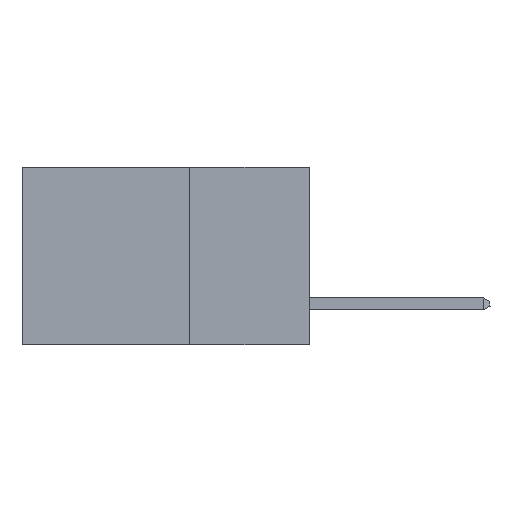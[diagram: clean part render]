
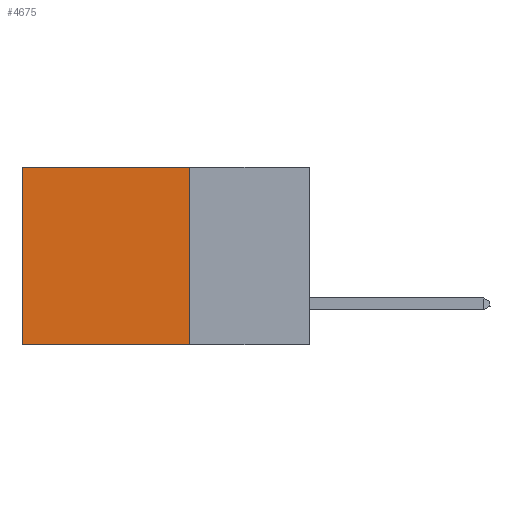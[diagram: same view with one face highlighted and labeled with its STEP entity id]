
A CAD part, left-side view. The second image highlights one B-rep face of the part: STEP entity #4675.
In plain terms, the highlighted planar face has unit normal (-1, 0, 0).
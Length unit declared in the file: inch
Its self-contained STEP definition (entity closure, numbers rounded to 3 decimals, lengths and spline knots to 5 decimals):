
#105 = EDGE_CURVE ( 'NONE', #2544, #1523, #12002, .T. ) ;
#323 = LINE ( 'NONE', #5854, #1986 ) ;
#518 = LINE ( 'NONE', #4223, #8856 ) ;
#544 = DIRECTION ( 'NONE',  ( 0., 1., 0. ) ) ;
#1337 = DIRECTION ( 'NONE',  ( 0., 0., -1. ) ) ;
#1523 = VERTEX_POINT ( 'NONE', #6386 ) ;
#1844 = EDGE_CURVE ( 'NONE', #1523, #12738, #323, .T. ) ;
#1986 = VECTOR ( 'NONE', #544, 39.37008 ) ;
#2349 = CARTESIAN_POINT ( 'NONE',  ( 0.2875, 0.25, 0. ) ) ;
#2544 = VERTEX_POINT ( 'NONE', #4369 ) ;
#2839 = CARTESIAN_POINT ( 'NONE',  ( 0.2875, 0.25, 0. ) ) ;
#3504 = VECTOR ( 'NONE', #5004, 39.37008 ) ;
#3887 = ORIENTED_EDGE ( 'NONE', *, *, #6979, .T. ) ;
#3894 = EDGE_LOOP ( 'NONE', ( #13096, #9598, #9846, #3887 ) ) ;
#4088 = CARTESIAN_POINT ( 'NONE',  ( 0.2875, 0.6, -0.37 ) ) ;
#4223 = CARTESIAN_POINT ( 'NONE',  ( 0.2875, 0.6, 0. ) ) ;
#4369 = CARTESIAN_POINT ( 'NONE',  ( 0.2875, 0.25, 0. ) ) ;
#4675 = ADVANCED_FACE ( 'NONE', ( #8425 ), #10251, .F. ) ;
#4723 = AXIS2_PLACEMENT_3D ( 'NONE', #2349, #9609, #1337 ) ;
#5004 = DIRECTION ( 'NONE',  ( 0., 0., -1. ) ) ;
#5277 = VERTEX_POINT ( 'NONE', #9862 ) ;
#5854 = CARTESIAN_POINT ( 'NONE',  ( 0.2875, 0.25, -0.37 ) ) ;
#6298 = DIRECTION ( 'NONE',  ( 0., 1., 0. ) ) ;
#6386 = CARTESIAN_POINT ( 'NONE',  ( 0.2875, 0.25, -0.37 ) ) ;
#6979 = EDGE_CURVE ( 'NONE', #2544, #5277, #13600, .T. ) ;
#8425 = FACE_OUTER_BOUND ( 'NONE', #3894, .T. ) ;
#8856 = VECTOR ( 'NONE', #12754, 39.37008 ) ;
#9598 = ORIENTED_EDGE ( 'NONE', *, *, #1844, .F. ) ;
#9609 = DIRECTION ( 'NONE',  ( 1., 0., 0. ) ) ;
#9846 = ORIENTED_EDGE ( 'NONE', *, *, #105, .F. ) ;
#9862 = CARTESIAN_POINT ( 'NONE',  ( 0.2875, 0.6, 0. ) ) ;
#10251 = PLANE ( 'NONE',  #4723 ) ;
#10469 = VECTOR ( 'NONE', #6298, 39.37008 ) ;
#11567 = CARTESIAN_POINT ( 'NONE',  ( 0.2875, 0.25, 0. ) ) ;
#12002 = LINE ( 'NONE', #2839, #3504 ) ;
#12065 = EDGE_CURVE ( 'NONE', #5277, #12738, #518, .T. ) ;
#12738 = VERTEX_POINT ( 'NONE', #4088 ) ;
#12754 = DIRECTION ( 'NONE',  ( 0., 0., -1. ) ) ;
#13096 = ORIENTED_EDGE ( 'NONE', *, *, #12065, .T. ) ;
#13600 = LINE ( 'NONE', #11567, #10469 ) ;
